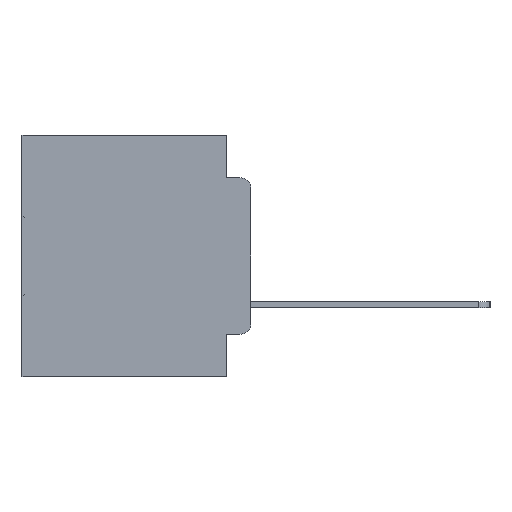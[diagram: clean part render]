
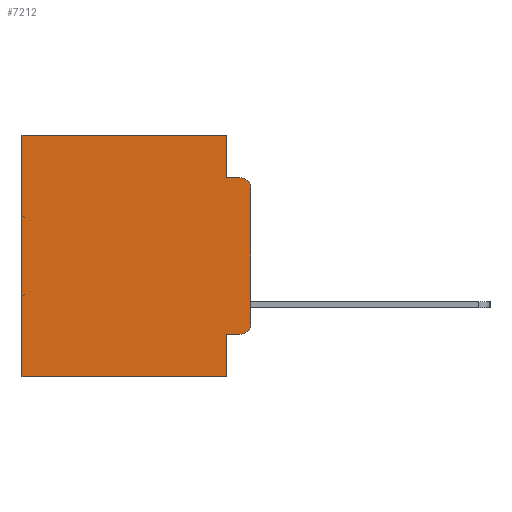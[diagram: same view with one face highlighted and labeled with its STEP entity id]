
A CAD part, left-side view. The second image highlights one B-rep face of the part: STEP entity #7212.
In plain terms, the highlighted planar face has unit normal (-1, 0, 0).
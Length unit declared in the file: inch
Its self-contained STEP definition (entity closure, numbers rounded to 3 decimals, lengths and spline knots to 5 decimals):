
#532 = DIRECTION ( 'NONE',  ( 0., 0., -1. ) ) ;
#900 = VERTEX_POINT ( 'NONE', #4744 ) ;
#1090 = CARTESIAN_POINT ( 'NONE',  ( 0.298, 0.051, 0. ) ) ;
#1672 = VECTOR ( 'NONE', #5500, 39.37008 ) ;
#2021 = ORIENTED_EDGE ( 'NONE', *, *, #10668, .F. ) ;
#2505 = LINE ( 'NONE', #9857, #3400 ) ;
#2582 = ORIENTED_EDGE ( 'NONE', *, *, #24033, .T. ) ;
#2970 = LINE ( 'NONE', #14105, #29078 ) ;
#3262 = PLANE ( 'NONE',  #4216 ) ;
#3400 = VECTOR ( 'NONE', #27346, 39.37008 ) ;
#3410 = VECTOR ( 'NONE', #17411, 39.37008 ) ;
#3426 = DIRECTION ( 'NONE',  ( 0., 0., -1. ) ) ;
#4216 = AXIS2_PLACEMENT_3D ( 'NONE', #11427, #14068, #30782 ) ;
#4682 = DIRECTION ( 'NONE',  ( 0., 0., -1. ) ) ;
#4744 = CARTESIAN_POINT ( 'NONE',  ( 0.298, 0.02, -0.4115 ) ) ;
#5487 = LINE ( 'NONE', #32046, #31067 ) ;
#5500 = DIRECTION ( 'NONE',  ( 0., 1., 0. ) ) ;
#5731 = VERTEX_POINT ( 'NONE', #23971 ) ;
#6037 = CARTESIAN_POINT ( 'NONE',  ( 0.298, 0.051, -0.5 ) ) ;
#7212 = ADVANCED_FACE ( 'NONE', ( #19249 ), #3262, .F. ) ;
#8857 = VECTOR ( 'NONE', #32584, 39.37008 ) ;
#8991 = LINE ( 'NONE', #13493, #1672 ) ;
#8998 = LINE ( 'NONE', #1090, #21891 ) ;
#9226 = CARTESIAN_POINT ( 'NONE',  ( 0.298, 0.02, -0.3915 ) ) ;
#9724 = LINE ( 'NONE', #18733, #8857 ) ;
#9857 = CARTESIAN_POINT ( 'NONE',  ( 0.298, 0.051, -0.4115 ) ) ;
#10668 = EDGE_CURVE ( 'NONE', #16686, #19222, #9724, .T. ) ;
#11075 = CARTESIAN_POINT ( 'NONE',  ( 0.298, 0.051, -0.0885 ) ) ;
#11427 = CARTESIAN_POINT ( 'NONE',  ( 0.298, 0., 0. ) ) ;
#11672 = ORIENTED_EDGE ( 'NONE', *, *, #16380, .F. ) ;
#11756 = VERTEX_POINT ( 'NONE', #27710 ) ;
#11910 = DIRECTION ( 'NONE',  ( 0., 0., -1. ) ) ;
#13007 = AXIS2_PLACEMENT_3D ( 'NONE', #30880, #16737, #532 ) ;
#13493 = CARTESIAN_POINT ( 'NONE',  ( 0.298, 0., 0. ) ) ;
#14068 = DIRECTION ( 'NONE',  ( 1., 0., 0. ) ) ;
#14105 = CARTESIAN_POINT ( 'NONE',  ( 0.298, 0.051, 0. ) ) ;
#14493 = ORIENTED_EDGE ( 'NONE', *, *, #17573, .F. ) ;
#14774 = LINE ( 'NONE', #25129, #27782 ) ;
#14893 = CARTESIAN_POINT ( 'NONE',  ( 0.298, 0.051, -0.0885 ) ) ;
#15711 = EDGE_CURVE ( 'NONE', #11756, #27505, #8998, .T. ) ;
#15947 = ORIENTED_EDGE ( 'NONE', *, *, #17432, .T. ) ;
#16106 = VERTEX_POINT ( 'NONE', #16635 ) ;
#16132 = EDGE_CURVE ( 'NONE', #16106, #5731, #28792, .T. ) ;
#16380 = EDGE_CURVE ( 'NONE', #16106, #16559, #14774, .T. ) ;
#16559 = VERTEX_POINT ( 'NONE', #28154 ) ;
#16635 = CARTESIAN_POINT ( 'NONE',  ( 0.298, 0., -0.1085 ) ) ;
#16686 = VERTEX_POINT ( 'NONE', #6037 ) ;
#16737 = DIRECTION ( 'NONE',  ( -1., 0., 0. ) ) ;
#16901 = EDGE_CURVE ( 'NONE', #23154, #900, #2505, .T. ) ;
#17043 = EDGE_CURVE ( 'NONE', #30076, #19222, #5487, .T. ) ;
#17340 = EDGE_CURVE ( 'NONE', #23154, #16686, #2970, .T. ) ;
#17411 = DIRECTION ( 'NONE',  ( 0., -1., 0. ) ) ;
#17432 = EDGE_CURVE ( 'NONE', #900, #16559, #27757, .T. ) ;
#17478 = LINE ( 'NONE', #14893, #3410 ) ;
#17573 = EDGE_CURVE ( 'NONE', #27505, #5731, #17478, .T. ) ;
#18733 = CARTESIAN_POINT ( 'NONE',  ( 0.298, 0., -0.5 ) ) ;
#18986 = ORIENTED_EDGE ( 'NONE', *, *, #16132, .T. ) ;
#19222 = VERTEX_POINT ( 'NONE', #24935 ) ;
#19249 = FACE_OUTER_BOUND ( 'NONE', #21872, .T. ) ;
#19588 = ORIENTED_EDGE ( 'NONE', *, *, #17340, .F. ) ;
#20692 = DIRECTION ( 'NONE',  ( 0., 0., -1. ) ) ;
#21605 = ORIENTED_EDGE ( 'NONE', *, *, #15711, .F. ) ;
#21856 = ORIENTED_EDGE ( 'NONE', *, *, #17043, .T. ) ;
#21872 = EDGE_LOOP ( 'NONE', ( #11672, #18986, #14493, #21605, #2582, #21856, #2021, #19588, #29627, #15947 ) ) ;
#21891 = VECTOR ( 'NONE', #22131, 39.37008 ) ;
#22131 = DIRECTION ( 'NONE',  ( 0., 0., -1. ) ) ;
#23154 = VERTEX_POINT ( 'NONE', #29700 ) ;
#23971 = CARTESIAN_POINT ( 'NONE',  ( 0.298, 0.02, -0.0885 ) ) ;
#24033 = EDGE_CURVE ( 'NONE', #11756, #30076, #8991, .T. ) ;
#24636 = AXIS2_PLACEMENT_3D ( 'NONE', #9226, #26810, #11910 ) ;
#24935 = CARTESIAN_POINT ( 'NONE',  ( 0.298, 0.473, -0.5 ) ) ;
#25129 = CARTESIAN_POINT ( 'NONE',  ( 0.298, 0., 0. ) ) ;
#26810 = DIRECTION ( 'NONE',  ( -1., 0., 0. ) ) ;
#27346 = DIRECTION ( 'NONE',  ( 0., -1., 0. ) ) ;
#27505 = VERTEX_POINT ( 'NONE', #11075 ) ;
#27710 = CARTESIAN_POINT ( 'NONE',  ( 0.298, 0.051, 0. ) ) ;
#27757 = CIRCLE ( 'NONE', #24636, 0.02 ) ;
#27782 = VECTOR ( 'NONE', #4682, 39.37008 ) ;
#28154 = CARTESIAN_POINT ( 'NONE',  ( 0.298, 0., -0.3915 ) ) ;
#28792 = CIRCLE ( 'NONE', #13007, 0.02 ) ;
#29078 = VECTOR ( 'NONE', #3426, 39.37008 ) ;
#29627 = ORIENTED_EDGE ( 'NONE', *, *, #16901, .T. ) ;
#29700 = CARTESIAN_POINT ( 'NONE',  ( 0.298, 0.051, -0.4115 ) ) ;
#30076 = VERTEX_POINT ( 'NONE', #31814 ) ;
#30782 = DIRECTION ( 'NONE',  ( 0., 0., -1. ) ) ;
#30880 = CARTESIAN_POINT ( 'NONE',  ( 0.298, 0.02, -0.1085 ) ) ;
#31067 = VECTOR ( 'NONE', #20692, 39.37008 ) ;
#31814 = CARTESIAN_POINT ( 'NONE',  ( 0.298, 0.473, 0. ) ) ;
#32046 = CARTESIAN_POINT ( 'NONE',  ( 0.298, 0.473, 0. ) ) ;
#32584 = DIRECTION ( 'NONE',  ( 0., 1., 0. ) ) ;
